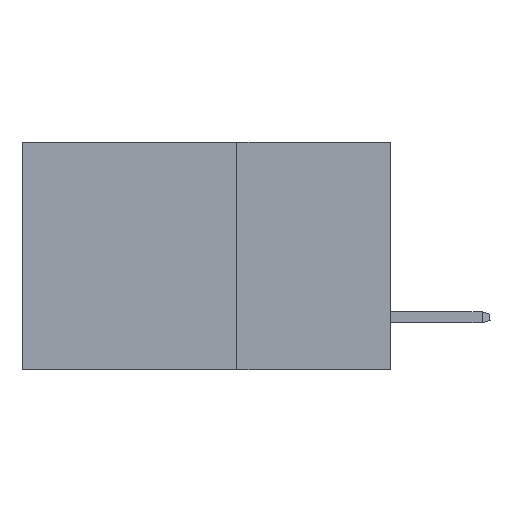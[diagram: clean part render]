
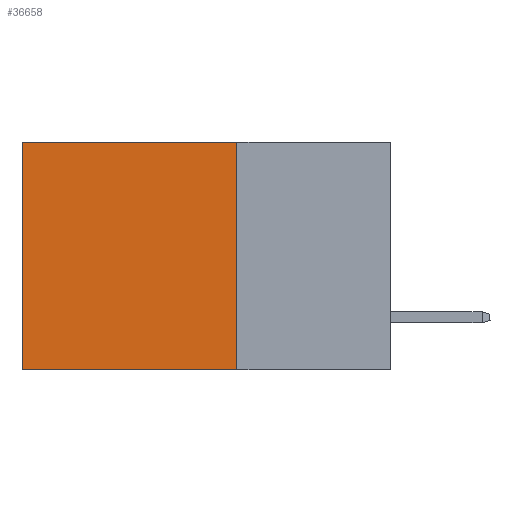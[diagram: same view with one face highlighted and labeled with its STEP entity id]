
A CAD part, left-side view. The second image highlights one B-rep face of the part: STEP entity #36658.
In plain terms, the highlighted planar face has unit normal (-1, 0, 0).
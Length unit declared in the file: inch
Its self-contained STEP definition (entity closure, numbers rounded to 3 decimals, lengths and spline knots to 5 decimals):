
#262 = EDGE_CURVE ( 'NONE', #30510, #410, #20228, .T. ) ;
#410 = VERTEX_POINT ( 'NONE', #8467 ) ;
#2992 = VECTOR ( 'NONE', #33879, 39.37008 ) ;
#3426 = DIRECTION ( 'NONE',  ( 0., 0., -1. ) ) ;
#4153 = ORIENTED_EDGE ( 'NONE', *, *, #24715, .F. ) ;
#5928 = LINE ( 'NONE', #30758, #2992 ) ;
#6848 = AXIS2_PLACEMENT_3D ( 'NONE', #28141, #22113, #3426 ) ;
#8201 = CARTESIAN_POINT ( 'NONE',  ( 0.2875, 0.25, 0. ) ) ;
#8250 = ORIENTED_EDGE ( 'NONE', *, *, #262, .F. ) ;
#8467 = CARTESIAN_POINT ( 'NONE',  ( 0.2875, 0.25, -0.37 ) ) ;
#9117 = EDGE_CURVE ( 'NONE', #10709, #20870, #19672, .T. ) ;
#10709 = VERTEX_POINT ( 'NONE', #29121 ) ;
#11149 = DIRECTION ( 'NONE',  ( 0., 0., -1. ) ) ;
#11636 = CARTESIAN_POINT ( 'NONE',  ( 0.2875, 0.25, 0. ) ) ;
#15418 = LINE ( 'NONE', #31384, #22186 ) ;
#19672 = LINE ( 'NONE', #20330, #25537 ) ;
#20228 = LINE ( 'NONE', #11636, #27095 ) ;
#20330 = CARTESIAN_POINT ( 'NONE',  ( 0.2875, 0.6, 0. ) ) ;
#20870 = VERTEX_POINT ( 'NONE', #20972 ) ;
#20972 = CARTESIAN_POINT ( 'NONE',  ( 0.2875, 0.6, -0.37 ) ) ;
#22113 = DIRECTION ( 'NONE',  ( 1., 0., 0. ) ) ;
#22186 = VECTOR ( 'NONE', #34509, 39.37008 ) ;
#24715 = EDGE_CURVE ( 'NONE', #410, #20870, #15418, .T. ) ;
#25537 = VECTOR ( 'NONE', #11149, 39.37008 ) ;
#25725 = FACE_OUTER_BOUND ( 'NONE', #32125, .T. ) ;
#27095 = VECTOR ( 'NONE', #33403, 39.37008 ) ;
#28141 = CARTESIAN_POINT ( 'NONE',  ( 0.2875, 0.25, 0. ) ) ;
#29121 = CARTESIAN_POINT ( 'NONE',  ( 0.2875, 0.6, 0. ) ) ;
#30510 = VERTEX_POINT ( 'NONE', #8201 ) ;
#30626 = EDGE_CURVE ( 'NONE', #30510, #10709, #5928, .T. ) ;
#30758 = CARTESIAN_POINT ( 'NONE',  ( 0.2875, 0.25, 0. ) ) ;
#31304 = PLANE ( 'NONE',  #6848 ) ;
#31384 = CARTESIAN_POINT ( 'NONE',  ( 0.2875, 0.25, -0.37 ) ) ;
#32125 = EDGE_LOOP ( 'NONE', ( #35193, #4153, #8250, #35255 ) ) ;
#33403 = DIRECTION ( 'NONE',  ( 0., 0., -1. ) ) ;
#33879 = DIRECTION ( 'NONE',  ( 0., 1., 0. ) ) ;
#34509 = DIRECTION ( 'NONE',  ( 0., 1., 0. ) ) ;
#35193 = ORIENTED_EDGE ( 'NONE', *, *, #9117, .T. ) ;
#35255 = ORIENTED_EDGE ( 'NONE', *, *, #30626, .T. ) ;
#36658 = ADVANCED_FACE ( 'NONE', ( #25725 ), #31304, .F. ) ;
